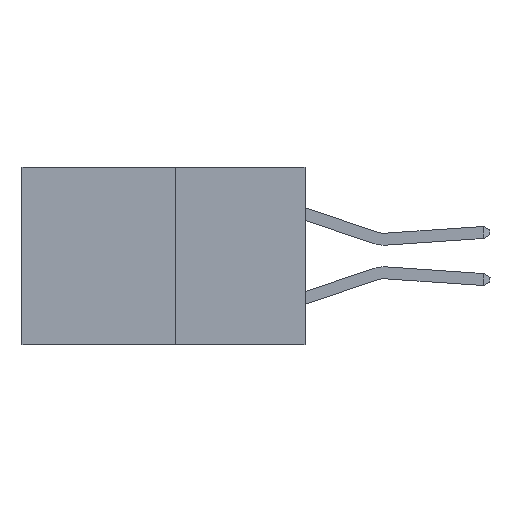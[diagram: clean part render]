
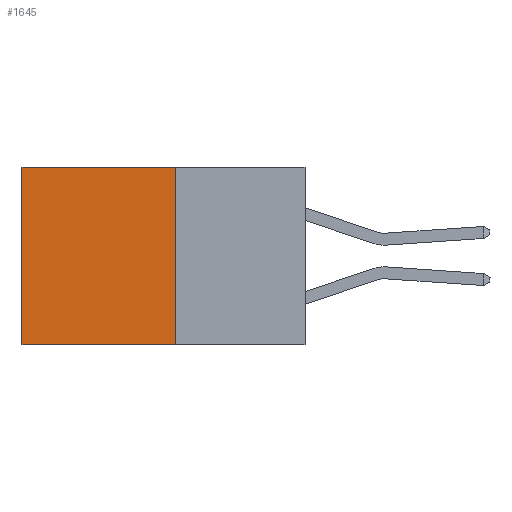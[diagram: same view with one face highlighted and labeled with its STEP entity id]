
A CAD part, left-side view. The second image highlights one B-rep face of the part: STEP entity #1645.
In plain terms, the highlighted planar face has unit normal (-1, 0, 0).
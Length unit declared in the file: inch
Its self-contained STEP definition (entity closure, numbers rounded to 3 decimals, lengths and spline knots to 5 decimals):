
#1180 = VECTOR ( 'NONE', #6489, 39.37008 ) ;
#1645 = ADVANCED_FACE ( 'NONE', ( #4131 ), #5391, .F. ) ;
#2497 = CARTESIAN_POINT ( 'NONE',  ( 0.277, 0.27, -0.37 ) ) ;
#2514 = ORIENTED_EDGE ( 'NONE', *, *, #4054, .F. ) ;
#2659 = VECTOR ( 'NONE', #5329, 39.37008 ) ;
#2723 = EDGE_CURVE ( 'NONE', #4267, #7192, #3221, .T. ) ;
#2886 = EDGE_CURVE ( 'NONE', #7192, #6579, #7298, .T. ) ;
#3221 = LINE ( 'NONE', #6454, #1180 ) ;
#3642 = AXIS2_PLACEMENT_3D ( 'NONE', #7067, #4305, #5113 ) ;
#3778 = EDGE_CURVE ( 'NONE', #4083, #6579, #4737, .T. ) ;
#4054 = EDGE_CURVE ( 'NONE', #4267, #4083, #5604, .T. ) ;
#4083 = VERTEX_POINT ( 'NONE', #7178 ) ;
#4128 = ORIENTED_EDGE ( 'NONE', *, *, #2723, .T. ) ;
#4131 = FACE_OUTER_BOUND ( 'NONE', #5454, .T. ) ;
#4267 = VERTEX_POINT ( 'NONE', #5046 ) ;
#4305 = DIRECTION ( 'NONE',  ( 1., 0., 0. ) ) ;
#4378 = CARTESIAN_POINT ( 'NONE',  ( 0.277, 0.59, -0.37 ) ) ;
#4656 = ORIENTED_EDGE ( 'NONE', *, *, #3778, .F. ) ;
#4737 = LINE ( 'NONE', #5704, #7343 ) ;
#4844 = CARTESIAN_POINT ( 'NONE',  ( 0.277, 0.59, 0. ) ) ;
#5046 = CARTESIAN_POINT ( 'NONE',  ( 0.277, 0.27, 0. ) ) ;
#5113 = DIRECTION ( 'NONE',  ( 0., 0., -1. ) ) ;
#5169 = DIRECTION ( 'NONE',  ( 0., 0., -1. ) ) ;
#5329 = DIRECTION ( 'NONE',  ( 0., 0., -1. ) ) ;
#5391 = PLANE ( 'NONE',  #3642 ) ;
#5454 = EDGE_LOOP ( 'NONE', ( #6114, #4656, #2514, #4128 ) ) ;
#5574 = CARTESIAN_POINT ( 'NONE',  ( 0.277, 0.59, -0.37 ) ) ;
#5604 = LINE ( 'NONE', #2497, #6842 ) ;
#5704 = CARTESIAN_POINT ( 'NONE',  ( 0.277, 0.27, -0.37 ) ) ;
#5748 = DIRECTION ( 'NONE',  ( 0., 1., 0. ) ) ;
#6114 = ORIENTED_EDGE ( 'NONE', *, *, #2886, .T. ) ;
#6454 = CARTESIAN_POINT ( 'NONE',  ( 0.277, 0.27, 0. ) ) ;
#6489 = DIRECTION ( 'NONE',  ( 0., 1., 0. ) ) ;
#6579 = VERTEX_POINT ( 'NONE', #5574 ) ;
#6842 = VECTOR ( 'NONE', #5169, 39.37008 ) ;
#7067 = CARTESIAN_POINT ( 'NONE',  ( 0.277, 0.27, -0.37 ) ) ;
#7178 = CARTESIAN_POINT ( 'NONE',  ( 0.277, 0.27, -0.37 ) ) ;
#7192 = VERTEX_POINT ( 'NONE', #4844 ) ;
#7298 = LINE ( 'NONE', #4378, #2659 ) ;
#7343 = VECTOR ( 'NONE', #5748, 39.37008 ) ;
